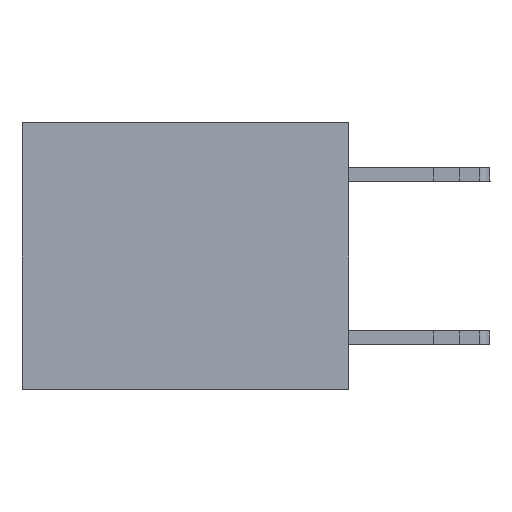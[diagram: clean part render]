
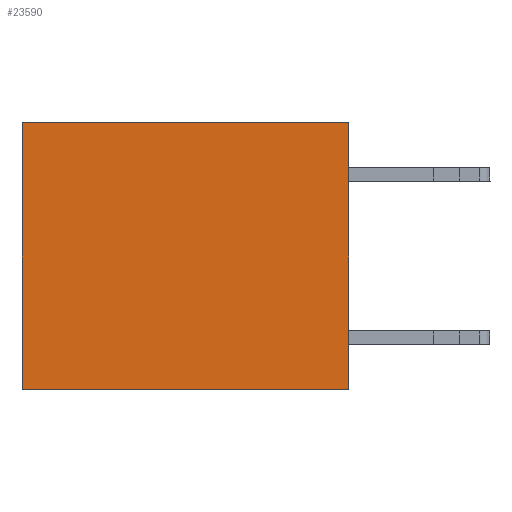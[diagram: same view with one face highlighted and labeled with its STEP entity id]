
A CAD part, left-side view. The second image highlights one B-rep face of the part: STEP entity #23590.
In plain terms, the highlighted planar face has unit normal (-1, 0, 0).
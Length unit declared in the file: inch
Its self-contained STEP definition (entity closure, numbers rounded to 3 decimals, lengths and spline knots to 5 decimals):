
#387 = DIRECTION ( 'NONE',  ( 0., 0., -1. ) ) ;
#484 = VERTEX_POINT ( 'NONE', #11694 ) ;
#776 = CARTESIAN_POINT ( 'NONE',  ( 0.3165, 0.6, -0.49 ) ) ;
#1360 = DIRECTION ( 'NONE',  ( 0., 1., 0. ) ) ;
#1496 = LINE ( 'NONE', #5048, #14401 ) ;
#2224 = ORIENTED_EDGE ( 'NONE', *, *, #22221, .F. ) ;
#2231 = VERTEX_POINT ( 'NONE', #14761 ) ;
#2319 = CARTESIAN_POINT ( 'NONE',  ( 0.3165, 0.6, 0. ) ) ;
#4383 = VERTEX_POINT ( 'NONE', #776 ) ;
#5048 = CARTESIAN_POINT ( 'NONE',  ( 0.3165, 0., -0.49 ) ) ;
#5137 = DIRECTION ( 'NONE',  ( 0., 0., -1. ) ) ;
#5965 = LINE ( 'NONE', #17004, #11758 ) ;
#7364 = EDGE_CURVE ( 'NONE', #2231, #25656, #22869, .T. ) ;
#8671 = PLANE ( 'NONE',  #12130 ) ;
#9309 = DIRECTION ( 'NONE',  ( 1., 0., 0. ) ) ;
#9522 = FACE_OUTER_BOUND ( 'NONE', #20135, .T. ) ;
#9937 = ORIENTED_EDGE ( 'NONE', *, *, #7364, .T. ) ;
#10920 = DIRECTION ( 'NONE',  ( 0., 0., -1. ) ) ;
#10931 = CARTESIAN_POINT ( 'NONE',  ( 0.3165, 0., -0.49 ) ) ;
#11694 = CARTESIAN_POINT ( 'NONE',  ( 0.3165, 0., -0.49 ) ) ;
#11758 = VECTOR ( 'NONE', #10920, 39.37008 ) ;
#12057 = CARTESIAN_POINT ( 'NONE',  ( 0.3165, 0., -0.49 ) ) ;
#12130 = AXIS2_PLACEMENT_3D ( 'NONE', #10931, #9309, #5137 ) ;
#14039 = ORIENTED_EDGE ( 'NONE', *, *, #23854, .F. ) ;
#14401 = VECTOR ( 'NONE', #15575, 39.37008 ) ;
#14761 = CARTESIAN_POINT ( 'NONE',  ( 0.3165, 0., 0. ) ) ;
#15575 = DIRECTION ( 'NONE',  ( 0., 1., 0. ) ) ;
#17004 = CARTESIAN_POINT ( 'NONE',  ( 0.3165, 0.6, -0.49 ) ) ;
#17438 = VECTOR ( 'NONE', #1360, 39.37008 ) ;
#18937 = EDGE_CURVE ( 'NONE', #25656, #4383, #5965, .T. ) ;
#20135 = EDGE_LOOP ( 'NONE', ( #20852, #2224, #14039, #9937 ) ) ;
#20852 = ORIENTED_EDGE ( 'NONE', *, *, #18937, .T. ) ;
#22221 = EDGE_CURVE ( 'NONE', #484, #4383, #1496, .T. ) ;
#22869 = LINE ( 'NONE', #23865, #17438 ) ;
#23590 = ADVANCED_FACE ( 'NONE', ( #9522 ), #8671, .F. ) ;
#23657 = LINE ( 'NONE', #12057, #25910 ) ;
#23854 = EDGE_CURVE ( 'NONE', #2231, #484, #23657, .T. ) ;
#23865 = CARTESIAN_POINT ( 'NONE',  ( 0.3165, 0., 0. ) ) ;
#25656 = VERTEX_POINT ( 'NONE', #2319 ) ;
#25910 = VECTOR ( 'NONE', #387, 39.37008 ) ;
